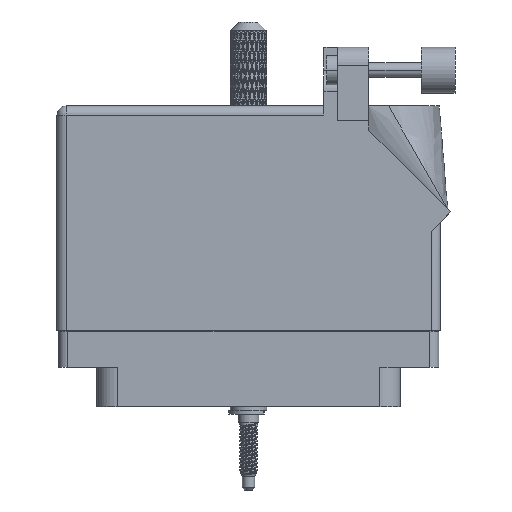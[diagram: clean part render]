
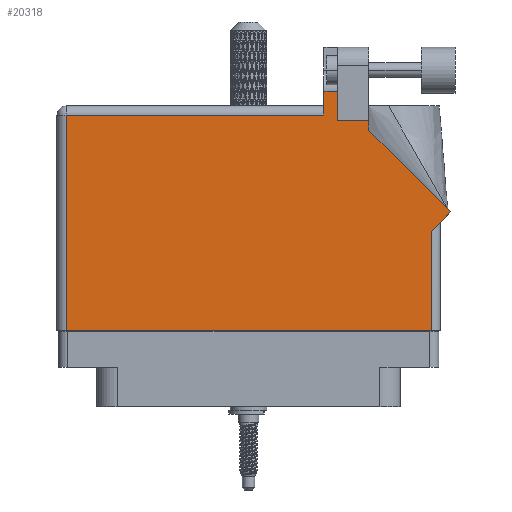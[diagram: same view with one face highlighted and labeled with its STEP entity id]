
A CAD part, front view. The second image highlights one B-rep face of the part: STEP entity #20318.
In plain terms, the highlighted face is planar.
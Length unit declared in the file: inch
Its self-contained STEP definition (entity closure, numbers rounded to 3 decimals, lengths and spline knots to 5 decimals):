
#4646 = CARTESIAN_POINT ( 'NONE',  ( -1.244, -0.1, 0.455 ) ) ;
#5091 = ORIENTED_EDGE ( 'NONE', *, *, #63513, .T. ) ;
#6780 = ORIENTED_EDGE ( 'NONE', *, *, #35369, .T. ) ;
#9205 = EDGE_CURVE ( 'NONE', #43345, #95197, #57301, .T. ) ;
#9315 = VECTOR ( 'NONE', #17450, 39.37008 ) ;
#9325 = VERTEX_POINT ( 'NONE', #27643 ) ;
#10641 = CARTESIAN_POINT ( 'NONE',  ( 0.513, 1.5315, 0.455 ) ) ;
#12496 = VECTOR ( 'NONE', #20168, 39.37008 ) ;
#13461 = ORIENTED_EDGE ( 'NONE', *, *, #106848, .T. ) ;
#13499 = CARTESIAN_POINT ( 'NONE',  ( 0.607, 1.33, 0.455 ) ) ;
#16551 = VECTOR ( 'NONE', #102526, 39.37008 ) ;
#17023 = CARTESIAN_POINT ( 'NONE',  ( 1.37671, 0.70771, 0.455 ) ) ;
#17088 = EDGE_CURVE ( 'NONE', #51630, #43891, #102494, .T. ) ;
#17450 = DIRECTION ( 'NONE',  ( 1., 0., 0. ) ) ;
#17997 = LINE ( 'NONE', #30406, #104394 ) ;
#20005 = CARTESIAN_POINT ( 'NONE',  ( 0.93777, 1.5315, 0.455 ) ) ;
#20168 = DIRECTION ( 'NONE',  ( -1., 0., 0. ) ) ;
#20318 = ADVANCED_FACE ( 'NONE', ( #73403 ), #24073, .F. ) ;
#21585 = CARTESIAN_POINT ( 'NONE',  ( -1.306, 1.368, 0.455 ) ) ;
#23991 = DIRECTION ( 'NONE',  ( 0., -1., 0. ) ) ;
#24073 = PLANE ( 'NONE',  #109775 ) ;
#25223 = DIRECTION ( 'NONE',  ( 0., 0., -1. ) ) ;
#27271 = CARTESIAN_POINT ( 'NONE',  ( 1.306, 0.637, 0.455 ) ) ;
#27337 = EDGE_CURVE ( 'NONE', #79595, #43345, #42721, .T. ) ;
#27643 = CARTESIAN_POINT ( 'NONE',  ( 1.244, -0.1, 0.455 ) ) ;
#28011 = VECTOR ( 'NONE', #37234, 39.37008 ) ;
#30406 = CARTESIAN_POINT ( 'NONE',  ( 1.244, 0.637, 0.455 ) ) ;
#30660 = CARTESIAN_POINT ( 'NONE',  ( 0.607, 1.5315, 0.455 ) ) ;
#32131 = DIRECTION ( 'NONE',  ( -0.707, 0.707, 0. ) ) ;
#35369 = EDGE_CURVE ( 'NONE', #9325, #73763, #17997, .T. ) ;
#37234 = DIRECTION ( 'NONE',  ( -1., 0., 0. ) ) ;
#37538 = DIRECTION ( 'NONE',  ( 0.707, 0.707, 0. ) ) ;
#37912 = ORIENTED_EDGE ( 'NONE', *, *, #62940, .T. ) ;
#42576 = VERTEX_POINT ( 'NONE', #104217 ) ;
#42721 = LINE ( 'NONE', #64559, #12496 ) ;
#43345 = VERTEX_POINT ( 'NONE', #72385 ) ;
#43891 = VERTEX_POINT ( 'NONE', #78286 ) ;
#44302 = VERTEX_POINT ( 'NONE', #4646 ) ;
#45790 = ORIENTED_EDGE ( 'NONE', *, *, #9205, .T. ) ;
#48031 = LINE ( 'NONE', #58573, #108359 ) ;
#48559 = ORIENTED_EDGE ( 'NONE', *, *, #80955, .T. ) ;
#51630 = VERTEX_POINT ( 'NONE', #10641 ) ;
#52026 = ORIENTED_EDGE ( 'NONE', *, *, #53139, .T. ) ;
#53139 = EDGE_CURVE ( 'NONE', #43891, #42576, #62968, .T. ) ;
#53407 = VECTOR ( 'NONE', #100042, 39.37008 ) ;
#56300 = VERTEX_POINT ( 'NONE', #17023 ) ;
#56995 = CARTESIAN_POINT ( 'NONE',  ( 1.244, 0.575, 0.455 ) ) ;
#57301 = LINE ( 'NONE', #13499, #92830 ) ;
#58573 = CARTESIAN_POINT ( 'NONE',  ( 1.37671, 0.70771, 0.455 ) ) ;
#58731 = VECTOR ( 'NONE', #37538, 39.37008 ) ;
#58882 = CARTESIAN_POINT ( 'NONE',  ( -1.306, 1.43, 0.455 ) ) ;
#59102 = LINE ( 'NONE', #67330, #16551 ) ;
#62302 = CARTESIAN_POINT ( 'NONE',  ( 0.82, 1.33, 0.455 ) ) ;
#62853 = EDGE_CURVE ( 'NONE', #42576, #44302, #59102, .T. ) ;
#62940 = EDGE_CURVE ( 'NONE', #56300, #77967, #48031, .T. ) ;
#62968 = LINE ( 'NONE', #21585, #53407 ) ;
#63513 = EDGE_CURVE ( 'NONE', #77967, #79595, #82137, .T. ) ;
#63560 = LINE ( 'NONE', #20005, #28011 ) ;
#64559 = CARTESIAN_POINT ( 'NONE',  ( 0.82, 1.33, 0.455 ) ) ;
#66819 = CARTESIAN_POINT ( 'NONE',  ( 0.513, 1.43, 0.455 ) ) ;
#67330 = CARTESIAN_POINT ( 'NONE',  ( -1.244, -0.1, 0.455 ) ) ;
#68223 = LINE ( 'NONE', #69961, #9315 ) ;
#69961 = CARTESIAN_POINT ( 'NONE',  ( -1.306, -0.1, 0.455 ) ) ;
#72385 = CARTESIAN_POINT ( 'NONE',  ( 0.607, 1.33, 0.455 ) ) ;
#72677 = VECTOR ( 'NONE', #79020, 39.37008 ) ;
#73403 = FACE_OUTER_BOUND ( 'NONE', #105293, .T. ) ;
#73763 = VERTEX_POINT ( 'NONE', #56995 ) ;
#76848 = ORIENTED_EDGE ( 'NONE', *, *, #17088, .T. ) ;
#77967 = VERTEX_POINT ( 'NONE', #94644 ) ;
#78286 = CARTESIAN_POINT ( 'NONE',  ( 0.513, 1.368, 0.455 ) ) ;
#79020 = DIRECTION ( 'NONE',  ( 0., 1., 0. ) ) ;
#79595 = VERTEX_POINT ( 'NONE', #62302 ) ;
#80482 = VECTOR ( 'NONE', #23991, 39.37008 ) ;
#80955 = EDGE_CURVE ( 'NONE', #95197, #51630, #63560, .T. ) ;
#82137 = LINE ( 'NONE', #89286, #72677 ) ;
#88278 = ORIENTED_EDGE ( 'NONE', *, *, #62853, .T. ) ;
#89286 = CARTESIAN_POINT ( 'NONE',  ( 0.82, 1.26442, 0.455 ) ) ;
#92284 = ORIENTED_EDGE ( 'NONE', *, *, #27337, .T. ) ;
#92830 = VECTOR ( 'NONE', #109214, 39.37008 ) ;
#92942 = LINE ( 'NONE', #27271, #58731 ) ;
#93664 = DIRECTION ( 'NONE',  ( -1., 0., 0. ) ) ;
#94644 = CARTESIAN_POINT ( 'NONE',  ( 0.82, 1.26442, 0.455 ) ) ;
#95197 = VERTEX_POINT ( 'NONE', #30660 ) ;
#99679 = DIRECTION ( 'NONE',  ( 0., 1., 0. ) ) ;
#100042 = DIRECTION ( 'NONE',  ( -1., 0., 0. ) ) ;
#102494 = LINE ( 'NONE', #66819, #80482 ) ;
#102526 = DIRECTION ( 'NONE',  ( 0., -1., 0. ) ) ;
#102883 = ORIENTED_EDGE ( 'NONE', *, *, #113048, .T. ) ;
#104217 = CARTESIAN_POINT ( 'NONE',  ( -1.244, 1.368, 0.455 ) ) ;
#104394 = VECTOR ( 'NONE', #99679, 39.37008 ) ;
#105293 = EDGE_LOOP ( 'NONE', ( #45790, #48559, #76848, #52026, #88278, #13461, #6780, #102883, #37912, #5091, #92284 ) ) ;
#106848 = EDGE_CURVE ( 'NONE', #44302, #9325, #68223, .T. ) ;
#108359 = VECTOR ( 'NONE', #32131, 39.37008 ) ;
#109214 = DIRECTION ( 'NONE',  ( 0., 1., 0. ) ) ;
#109775 = AXIS2_PLACEMENT_3D ( 'NONE', #58882, #25223, #93664 ) ;
#113048 = EDGE_CURVE ( 'NONE', #73763, #56300, #92942, .T. ) ;
